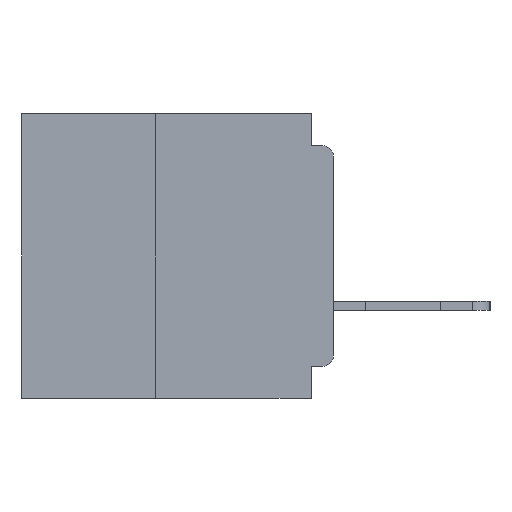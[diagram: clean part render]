
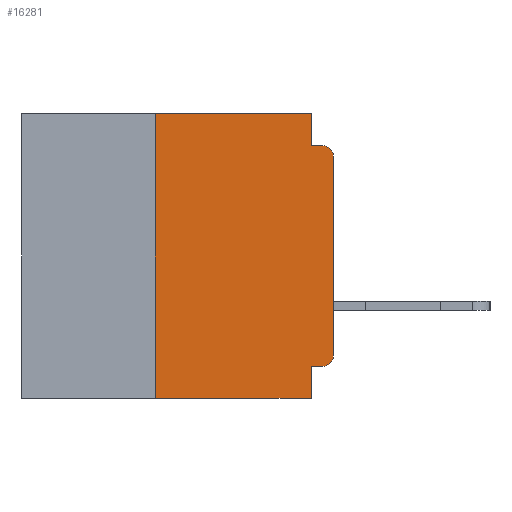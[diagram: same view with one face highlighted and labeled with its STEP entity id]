
A CAD part, left-side view. The second image highlights one B-rep face of the part: STEP entity #16281.
In plain terms, the highlighted planar face has unit normal (-1, 0, 0).
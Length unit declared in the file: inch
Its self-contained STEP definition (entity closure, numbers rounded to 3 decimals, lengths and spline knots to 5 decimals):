
#98 = ORIENTED_EDGE ( 'NONE', *, *, #22478, .F. ) ;
#555 = ORIENTED_EDGE ( 'NONE', *, *, #14313, .T. ) ;
#1007 = CIRCLE ( 'NONE', #9976, 0.015 ) ;
#1857 = VERTEX_POINT ( 'NONE', #6492 ) ;
#1865 = CARTESIAN_POINT ( 'NONE',  ( 0., 0.25, -0.4 ) ) ;
#2470 = VERTEX_POINT ( 'NONE', #15063 ) ;
#2728 = CARTESIAN_POINT ( 'NONE',  ( 0., 0.437, -0.4 ) ) ;
#2784 = DIRECTION ( 'NONE',  ( 0., 0., -1. ) ) ;
#3339 = ORIENTED_EDGE ( 'NONE', *, *, #7036, .F. ) ;
#3406 = CARTESIAN_POINT ( 'NONE',  ( 0., 0., -0.06 ) ) ;
#3436 = VECTOR ( 'NONE', #25152, 39.37008 ) ;
#3522 = VERTEX_POINT ( 'NONE', #37050 ) ;
#3874 = CIRCLE ( 'NONE', #11870, 0.015 ) ;
#3883 = EDGE_CURVE ( 'NONE', #6128, #12010, #28105, .T. ) ;
#3911 = EDGE_CURVE ( 'NONE', #3522, #2470, #4404, .T. ) ;
#3976 = DIRECTION ( 'NONE',  ( 0., 0., -1. ) ) ;
#4173 = FACE_OUTER_BOUND ( 'NONE', #7756, .T. ) ;
#4371 = EDGE_CURVE ( 'NONE', #27999, #3522, #19620, .T. ) ;
#4404 = LINE ( 'NONE', #32646, #27215 ) ;
#4780 = ORIENTED_EDGE ( 'NONE', *, *, #3911, .F. ) ;
#5010 = CARTESIAN_POINT ( 'NONE',  ( 0., 0.031, -0.355 ) ) ;
#5181 = CARTESIAN_POINT ( 'NONE',  ( 0., 0., -0.355 ) ) ;
#5187 = LINE ( 'NONE', #36686, #34665 ) ;
#5344 = DIRECTION ( 'NONE',  ( -1., 0., 0. ) ) ;
#5358 = DIRECTION ( 'NONE',  ( 0., 0., -1. ) ) ;
#5439 = CARTESIAN_POINT ( 'NONE',  ( 0., 0.25, 0. ) ) ;
#5548 = LINE ( 'NONE', #29543, #33255 ) ;
#5756 = VERTEX_POINT ( 'NONE', #26490 ) ;
#6128 = VERTEX_POINT ( 'NONE', #17138 ) ;
#6492 = CARTESIAN_POINT ( 'NONE',  ( 0., 0.015, -0.045 ) ) ;
#6538 = ORIENTED_EDGE ( 'NONE', *, *, #3883, .T. ) ;
#6696 = DIRECTION ( 'NONE',  ( 0., 0., 1. ) ) ;
#6892 = AXIS2_PLACEMENT_3D ( 'NONE', #8473, #19978, #2784 ) ;
#7036 = EDGE_CURVE ( 'NONE', #2470, #1857, #24814, .T. ) ;
#7756 = EDGE_LOOP ( 'NONE', ( #6538, #35532, #3339, #4780, #29402, #9402, #16592, #8537, #98, #555 ) ) ;
#8473 = CARTESIAN_POINT ( 'NONE',  ( 0., 0.437, 0. ) ) ;
#8537 = ORIENTED_EDGE ( 'NONE', *, *, #11808, .F. ) ;
#8631 = DIRECTION ( 'NONE',  ( -1., 0., 0. ) ) ;
#9000 = DIRECTION ( 'NONE',  ( 0., -1., 0. ) ) ;
#9402 = ORIENTED_EDGE ( 'NONE', *, *, #12863, .F. ) ;
#9459 = DIRECTION ( 'NONE',  ( 0., -1., 0. ) ) ;
#9976 = AXIS2_PLACEMENT_3D ( 'NONE', #25706, #8631, #28587 ) ;
#10211 = VECTOR ( 'NONE', #9000, 39.37008 ) ;
#11101 = LINE ( 'NONE', #5181, #3436 ) ;
#11120 = VERTEX_POINT ( 'NONE', #36481 ) ;
#11808 = EDGE_CURVE ( 'NONE', #17385, #11120, #5187, .T. ) ;
#11870 = AXIS2_PLACEMENT_3D ( 'NONE', #22480, #5344, #25305 ) ;
#12010 = VERTEX_POINT ( 'NONE', #3406 ) ;
#12298 = VERTEX_POINT ( 'NONE', #1865 ) ;
#12606 = DIRECTION ( 'NONE',  ( 0., 0., 1. ) ) ;
#12863 = EDGE_CURVE ( 'NONE', #12298, #27999, #5548, .T. ) ;
#14313 = EDGE_CURVE ( 'NONE', #5756, #6128, #3874, .T. ) ;
#15063 = CARTESIAN_POINT ( 'NONE',  ( 0., 0.031, -0.045 ) ) ;
#16281 = ADVANCED_FACE ( 'NONE', ( #4173 ), #37038, .F. ) ;
#16592 = ORIENTED_EDGE ( 'NONE', *, *, #30919, .T. ) ;
#17138 = CARTESIAN_POINT ( 'NONE',  ( 0., 0., -0.34 ) ) ;
#17385 = VERTEX_POINT ( 'NONE', #5010 ) ;
#17496 = CARTESIAN_POINT ( 'NONE',  ( 0., 0.437, 0. ) ) ;
#17954 = CARTESIAN_POINT ( 'NONE',  ( 0., 0., -0.045 ) ) ;
#19045 = VECTOR ( 'NONE', #34260, 39.37008 ) ;
#19620 = LINE ( 'NONE', #17496, #10211 ) ;
#19978 = DIRECTION ( 'NONE',  ( 1., 0., 0. ) ) ;
#22478 = EDGE_CURVE ( 'NONE', #5756, #17385, #11101, .T. ) ;
#22480 = CARTESIAN_POINT ( 'NONE',  ( 0., 0.015, -0.34 ) ) ;
#23941 = VECTOR ( 'NONE', #9459, 39.37008 ) ;
#24472 = EDGE_CURVE ( 'NONE', #12010, #1857, #1007, .T. ) ;
#24814 = LINE ( 'NONE', #17954, #23941 ) ;
#25152 = DIRECTION ( 'NONE',  ( 0., 1., 0. ) ) ;
#25305 = DIRECTION ( 'NONE',  ( 0., 0., -1. ) ) ;
#25706 = CARTESIAN_POINT ( 'NONE',  ( 0., 0.015, -0.06 ) ) ;
#26490 = CARTESIAN_POINT ( 'NONE',  ( 0., 0.015, -0.355 ) ) ;
#26861 = CARTESIAN_POINT ( 'NONE',  ( 0., 0., 0. ) ) ;
#27215 = VECTOR ( 'NONE', #3976, 39.37008 ) ;
#27999 = VERTEX_POINT ( 'NONE', #5439 ) ;
#28105 = LINE ( 'NONE', #26861, #33930 ) ;
#28587 = DIRECTION ( 'NONE',  ( 0., 0., -1. ) ) ;
#29402 = ORIENTED_EDGE ( 'NONE', *, *, #4371, .F. ) ;
#29543 = CARTESIAN_POINT ( 'NONE',  ( 0., 0.25, -0.4 ) ) ;
#30919 = EDGE_CURVE ( 'NONE', #12298, #11120, #35114, .T. ) ;
#32646 = CARTESIAN_POINT ( 'NONE',  ( 0., 0.031, 0. ) ) ;
#33255 = VECTOR ( 'NONE', #6696, 39.37008 ) ;
#33930 = VECTOR ( 'NONE', #12606, 39.37008 ) ;
#34260 = DIRECTION ( 'NONE',  ( 0., -1., 0. ) ) ;
#34665 = VECTOR ( 'NONE', #5358, 39.37008 ) ;
#35114 = LINE ( 'NONE', #2728, #19045 ) ;
#35532 = ORIENTED_EDGE ( 'NONE', *, *, #24472, .T. ) ;
#36481 = CARTESIAN_POINT ( 'NONE',  ( 0., 0.031, -0.4 ) ) ;
#36686 = CARTESIAN_POINT ( 'NONE',  ( 0., 0.031, -0.4 ) ) ;
#37038 = PLANE ( 'NONE',  #6892 ) ;
#37050 = CARTESIAN_POINT ( 'NONE',  ( 0., 0.031, 0. ) ) ;
